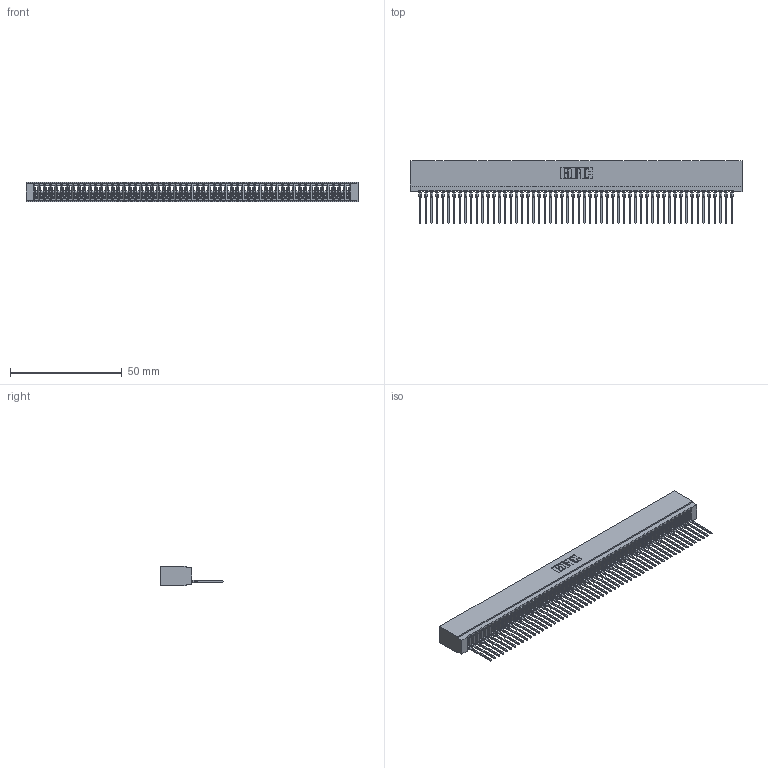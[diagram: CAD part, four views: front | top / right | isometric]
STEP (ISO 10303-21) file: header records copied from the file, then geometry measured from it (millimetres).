
FILE_DESCRIPTION (( 'STEP AP203' ), '1' );
FILE_NAME ('725-056-540-101.STEP', '2026-03-05T23:51:33', ( '' ), ( '' ), 'SwSTEP 2.0', 'SolidWorks 2023', '' );
FILE_SCHEMA (( 'CONFIG_CONTROL_DESIGN' ));
Length unit declared in the file: millimetre
Products named in the file (3): 725-056-540-101; 745-292-001_540; 725 Part_Insulator Option - 01
Assembly tree (57 placements, depth 2):
  725-056-540-101
    725 Part_Insulator Option - 01
    745-292-001_540  x56
Bounding box: 148.84 x 28.21 x 8.89 mm (x, y, z)
Volume: 11349.8 mm3; surface area: 22709 mm2
Topology: 57 solids, 57 shells, 6367 faces, 17502 edges, 11032 vertices
Faces by surface type: plane 3807, bspline 1120, cylinder 1104, torus 336
Entity records: 90538 total; most frequent: CARTESIAN_POINT 16455, ORIENTED_EDGE 15974, DIRECTION 13833, EDGE_CURVE 7987, VECTOR 7469, LINE 7469, VERTEX_POINT 5092, AXIS2_PLACEMENT_3D 3182
